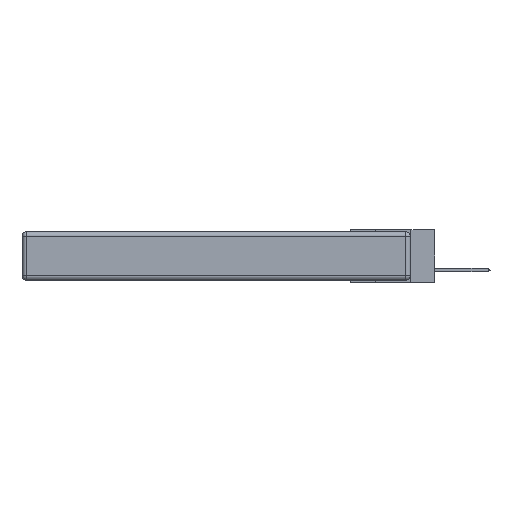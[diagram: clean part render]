
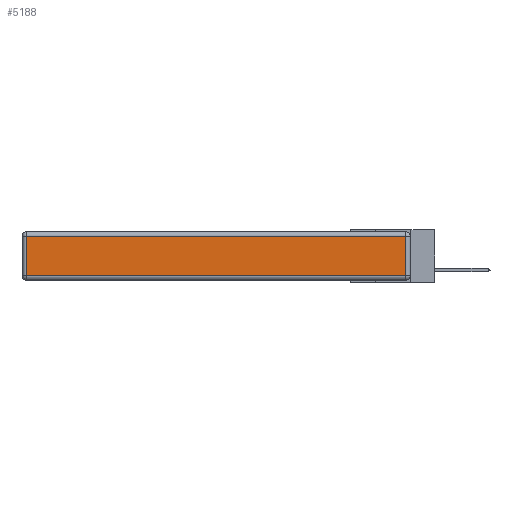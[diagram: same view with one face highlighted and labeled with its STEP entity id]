
A CAD part, left-side view. The second image highlights one B-rep face of the part: STEP entity #5188.
In plain terms, the highlighted planar face has unit normal (-1, 0, 0).
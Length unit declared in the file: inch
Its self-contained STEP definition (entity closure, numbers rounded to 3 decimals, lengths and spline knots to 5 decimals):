
#80 = DIRECTION ( 'NONE',  ( 0., 0., 1. ) ) ;
#244 = VECTOR ( 'NONE', #6175, 39.37008 ) ;
#793 = CARTESIAN_POINT ( 'NONE',  ( 0., 0.03, -0.313 ) ) ;
#987 = DIRECTION ( 'NONE',  ( -1., 0., 0. ) ) ;
#1018 = CARTESIAN_POINT ( 'NONE',  ( 0., 2.72, -0.343 ) ) ;
#1278 = DIRECTION ( 'NONE',  ( 0., 0., -1. ) ) ;
#2064 = EDGE_CURVE ( 'NONE', #18340, #3528, #3497, .T. ) ;
#2160 = VECTOR ( 'NONE', #80, 39.37008 ) ;
#2346 = CARTESIAN_POINT ( 'NONE',  ( 0., 2.72, -0.313 ) ) ;
#2681 = PLANE ( 'NONE',  #8892 ) ;
#3001 = ORIENTED_EDGE ( 'NONE', *, *, #6426, .T. ) ;
#3497 = LINE ( 'NONE', #15521, #244 ) ;
#3528 = VERTEX_POINT ( 'NONE', #5087 ) ;
#4617 = DIRECTION ( 'NONE',  ( 0., 0., 1. ) ) ;
#5087 = CARTESIAN_POINT ( 'NONE',  ( 0., 2.72, -0.03 ) ) ;
#5188 = ADVANCED_FACE ( 'NONE', ( #19464 ), #2681, .T. ) ;
#5667 = CARTESIAN_POINT ( 'NONE',  ( 0., 0.03, -0.343 ) ) ;
#6175 = DIRECTION ( 'NONE',  ( 0., 1., 0. ) ) ;
#6426 = EDGE_CURVE ( 'NONE', #9684, #16796, #10391, .T. ) ;
#8892 = AXIS2_PLACEMENT_3D ( 'NONE', #15855, #987, #4617 ) ;
#9214 = VECTOR ( 'NONE', #20528, 39.37008 ) ;
#9684 = VERTEX_POINT ( 'NONE', #2346 ) ;
#10062 = LINE ( 'NONE', #5667, #2160 ) ;
#10391 = LINE ( 'NONE', #13003, #9214 ) ;
#10483 = EDGE_CURVE ( 'NONE', #3528, #9684, #23975, .T. ) ;
#13003 = CARTESIAN_POINT ( 'NONE',  ( 0., 0., -0.313 ) ) ;
#13748 = EDGE_LOOP ( 'NONE', ( #3001, #20335, #16811, #14951 ) ) ;
#14003 = VECTOR ( 'NONE', #1278, 39.37008 ) ;
#14951 = ORIENTED_EDGE ( 'NONE', *, *, #10483, .T. ) ;
#15175 = CARTESIAN_POINT ( 'NONE',  ( 0., 0.03, -0.03 ) ) ;
#15521 = CARTESIAN_POINT ( 'NONE',  ( 0., 2.75, -0.03 ) ) ;
#15855 = CARTESIAN_POINT ( 'NONE',  ( 0., 0., -0.343 ) ) ;
#16796 = VERTEX_POINT ( 'NONE', #793 ) ;
#16811 = ORIENTED_EDGE ( 'NONE', *, *, #2064, .T. ) ;
#18340 = VERTEX_POINT ( 'NONE', #15175 ) ;
#19464 = FACE_OUTER_BOUND ( 'NONE', #13748, .T. ) ;
#20335 = ORIENTED_EDGE ( 'NONE', *, *, #23713, .T. ) ;
#20528 = DIRECTION ( 'NONE',  ( 0., -1., 0. ) ) ;
#23713 = EDGE_CURVE ( 'NONE', #16796, #18340, #10062, .T. ) ;
#23975 = LINE ( 'NONE', #1018, #14003 ) ;
